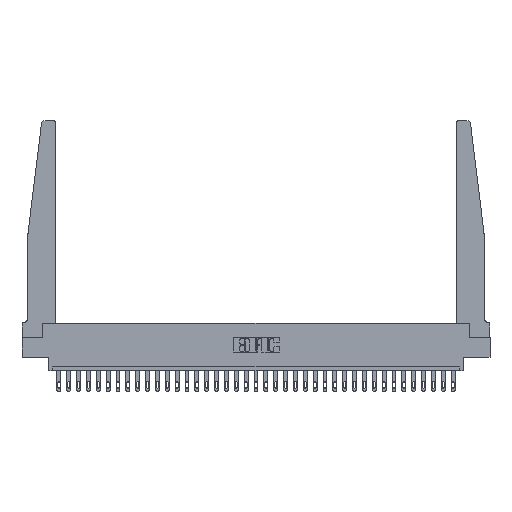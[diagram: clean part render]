
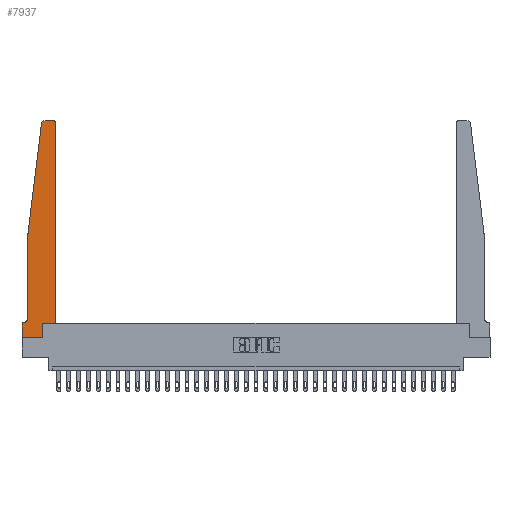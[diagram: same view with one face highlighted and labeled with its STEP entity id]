
A CAD part, top view. The second image highlights one B-rep face of the part: STEP entity #7937.
In plain terms, the highlighted planar face has unit normal (0, 0, 1).
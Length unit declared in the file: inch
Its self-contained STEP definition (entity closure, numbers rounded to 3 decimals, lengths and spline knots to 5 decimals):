
#10 = LINE ( 'NONE', #13769, #247 ) ;
#92 = DIRECTION ( 'NONE',  ( 1., 0., 0. ) ) ;
#103 = LINE ( 'NONE', #4939, #19569 ) ;
#247 = VECTOR ( 'NONE', #9384, 39.37008 ) ;
#401 = CARTESIAN_POINT ( 'NONE',  ( 0., 0.1875, 0.37 ) ) ;
#1106 = VERTEX_POINT ( 'NONE', #29358 ) ;
#1212 = ORIENTED_EDGE ( 'NONE', *, *, #13531, .T. ) ;
#1813 = VERTEX_POINT ( 'NONE', #18830 ) ;
#2293 = FACE_OUTER_BOUND ( 'NONE', #19335, .T. ) ;
#2329 = DIRECTION ( 'NONE',  ( -1., 0., 0. ) ) ;
#2357 = VERTEX_POINT ( 'NONE', #26692 ) ;
#2729 = DIRECTION ( 'NONE',  ( 0., 0., 1. ) ) ;
#2940 = VERTEX_POINT ( 'NONE', #24924 ) ;
#3674 = LINE ( 'NONE', #18184, #15856 ) ;
#3904 = CARTESIAN_POINT ( 'NONE',  ( 0.065, 1.25, 0.37 ) ) ;
#3967 = EDGE_CURVE ( 'NONE', #2940, #1813, #29030, .T. ) ;
#4042 = VECTOR ( 'NONE', #6650, 39.37008 ) ;
#4383 = EDGE_CURVE ( 'NONE', #9635, #28857, #103, .T. ) ;
#4545 = ORIENTED_EDGE ( 'NONE', *, *, #13422, .T. ) ;
#4939 = CARTESIAN_POINT ( 'NONE',  ( 0., 0., 0.37 ) ) ;
#5403 = LINE ( 'NONE', #29280, #7797 ) ;
#5461 = LINE ( 'NONE', #29186, #5809 ) ;
#5809 = VECTOR ( 'NONE', #27000, 39.37008 ) ;
#5812 = VERTEX_POINT ( 'NONE', #6454 ) ;
#6262 = ORIENTED_EDGE ( 'NONE', *, *, #21996, .T. ) ;
#6454 = CARTESIAN_POINT ( 'NONE',  ( 0.015, 0.1875, 0.37 ) ) ;
#6650 = DIRECTION ( 'NONE',  ( 0., 1., 0. ) ) ;
#7498 = DIRECTION ( 'NONE',  ( 0., 0., -1. ) ) ;
#7726 = LINE ( 'NONE', #17232, #14847 ) ;
#7797 = VECTOR ( 'NONE', #22091, 39.37008 ) ;
#7937 = ADVANCED_FACE ( 'NONE', ( #2293 ), #14307, .T. ) ;
#8455 = DIRECTION ( 'NONE',  ( 1., 0., 0. ) ) ;
#8988 = EDGE_CURVE ( 'NONE', #5812, #23784, #5461, .T. ) ;
#9278 = AXIS2_PLACEMENT_3D ( 'NONE', #401, #2729, #92 ) ;
#9384 = DIRECTION ( 'NONE',  ( 0., -1., 0. ) ) ;
#9620 = CARTESIAN_POINT ( 'NONE',  ( 0., 0., 0.37 ) ) ;
#9635 = VERTEX_POINT ( 'NONE', #9620 ) ;
#9976 = CARTESIAN_POINT ( 'NONE',  ( 0.015, 0.2375, 0.37 ) ) ;
#10148 = DIRECTION ( 'NONE',  ( 1., 0., 0. ) ) ;
#10258 = ORIENTED_EDGE ( 'NONE', *, *, #26736, .T. ) ;
#10427 = VERTEX_POINT ( 'NONE', #28549 ) ;
#10448 = ORIENTED_EDGE ( 'NONE', *, *, #3967, .T. ) ;
#10790 = CARTESIAN_POINT ( 'NONE',  ( 0.27653, 2.72, 0.37 ) ) ;
#12201 = ORIENTED_EDGE ( 'NONE', *, *, #4383, .T. ) ;
#12668 = VERTEX_POINT ( 'NONE', #15807 ) ;
#13422 = EDGE_CURVE ( 'NONE', #23784, #9635, #10, .T. ) ;
#13514 = CARTESIAN_POINT ( 'NONE',  ( 0.425, 0.18, 0.37 ) ) ;
#13531 = EDGE_CURVE ( 'NONE', #1106, #5812, #27179, .T. ) ;
#13600 = ORIENTED_EDGE ( 'NONE', *, *, #23601, .T. ) ;
#13769 = CARTESIAN_POINT ( 'NONE',  ( 0., 0., 0.37 ) ) ;
#13875 = EDGE_CURVE ( 'NONE', #1813, #23651, #23681, .T. ) ;
#14013 = DIRECTION ( 'NONE',  ( 1., 0., 0. ) ) ;
#14192 = CARTESIAN_POINT ( 'NONE',  ( 0.25, 2.75, 0.37 ) ) ;
#14307 = PLANE ( 'NONE',  #9278 ) ;
#14679 = VECTOR ( 'NONE', #2329, 39.37008 ) ;
#14847 = VECTOR ( 'NONE', #17072, 39.37008 ) ;
#14982 = CIRCLE ( 'NONE', #29922, 0.03 ) ;
#15807 = CARTESIAN_POINT ( 'NONE',  ( 0.2605, 0.18, 0.37 ) ) ;
#15856 = VECTOR ( 'NONE', #20822, 39.37008 ) ;
#16469 = VECTOR ( 'NONE', #17798, 39.37008 ) ;
#16712 = DIRECTION ( 'NONE',  ( 0., 0., 1. ) ) ;
#17072 = DIRECTION ( 'NONE',  ( 0., 1., 0. ) ) ;
#17232 = CARTESIAN_POINT ( 'NONE',  ( 0.2605, 0.18, 0.37 ) ) ;
#17532 = CARTESIAN_POINT ( 'NONE',  ( 0.27653, 2.75, 0.37 ) ) ;
#17798 = DIRECTION ( 'NONE',  ( 0., -1., 0. ) ) ;
#18184 = CARTESIAN_POINT ( 'NONE',  ( 0.425, 0.18, 0.37 ) ) ;
#18232 = ORIENTED_EDGE ( 'NONE', *, *, #27138, .T. ) ;
#18830 = CARTESIAN_POINT ( 'NONE',  ( 0.395, 2.75, 0.37 ) ) ;
#19335 = EDGE_LOOP ( 'NONE', ( #25082, #10258, #6262, #27633, #1212, #28051, #4545, #12201, #13600, #23103, #18232, #10448 ) ) ;
#19569 = VECTOR ( 'NONE', #14013, 39.37008 ) ;
#20822 = DIRECTION ( 'NONE',  ( 1., 0., 0. ) ) ;
#21899 = VERTEX_POINT ( 'NONE', #26937 ) ;
#21996 = EDGE_CURVE ( 'NONE', #21899, #10427, #5403, .T. ) ;
#22091 = DIRECTION ( 'NONE',  ( -0.122, -0.992, 0. ) ) ;
#22180 = EDGE_CURVE ( 'NONE', #12668, #2357, #3674, .T. ) ;
#22565 = AXIS2_PLACEMENT_3D ( 'NONE', #24332, #16712, #10148 ) ;
#23103 = ORIENTED_EDGE ( 'NONE', *, *, #22180, .T. ) ;
#23131 = CARTESIAN_POINT ( 'NONE',  ( 0., 0.1875, 0.37 ) ) ;
#23601 = EDGE_CURVE ( 'NONE', #28857, #12668, #7726, .T. ) ;
#23651 = VERTEX_POINT ( 'NONE', #17532 ) ;
#23681 = LINE ( 'NONE', #14192, #14679 ) ;
#23784 = VERTEX_POINT ( 'NONE', #23131 ) ;
#24332 = CARTESIAN_POINT ( 'NONE',  ( 0.395, 2.72, 0.37 ) ) ;
#24639 = DIRECTION ( 'NONE',  ( -1., 0., 0. ) ) ;
#24924 = CARTESIAN_POINT ( 'NONE',  ( 0.425, 2.72, 0.37 ) ) ;
#25082 = ORIENTED_EDGE ( 'NONE', *, *, #13875, .T. ) ;
#26692 = CARTESIAN_POINT ( 'NONE',  ( 0.425, 0.18, 0.37 ) ) ;
#26736 = EDGE_CURVE ( 'NONE', #23651, #21899, #14982, .T. ) ;
#26743 = EDGE_CURVE ( 'NONE', #10427, #1106, #27333, .T. ) ;
#26937 = CARTESIAN_POINT ( 'NONE',  ( 0.24675, 2.72367, 0.37 ) ) ;
#27000 = DIRECTION ( 'NONE',  ( -1., 0., 0. ) ) ;
#27138 = EDGE_CURVE ( 'NONE', #2357, #2940, #29626, .T. ) ;
#27179 = CIRCLE ( 'NONE', #30680, 0.05 ) ;
#27333 = LINE ( 'NONE', #3904, #16469 ) ;
#27633 = ORIENTED_EDGE ( 'NONE', *, *, #26743, .T. ) ;
#28051 = ORIENTED_EDGE ( 'NONE', *, *, #8988, .T. ) ;
#28549 = CARTESIAN_POINT ( 'NONE',  ( 0.065, 1.25, 0.37 ) ) ;
#28857 = VERTEX_POINT ( 'NONE', #30687 ) ;
#29030 = CIRCLE ( 'NONE', #22565, 0.03 ) ;
#29186 = CARTESIAN_POINT ( 'NONE',  ( 0.065, 0.1875, 0.37 ) ) ;
#29280 = CARTESIAN_POINT ( 'NONE',  ( 0.065, 1.25, 0.37 ) ) ;
#29358 = CARTESIAN_POINT ( 'NONE',  ( 0.065, 0.2375, 0.37 ) ) ;
#29626 = LINE ( 'NONE', #13514, #4042 ) ;
#29922 = AXIS2_PLACEMENT_3D ( 'NONE', #10790, #30125, #8455 ) ;
#30125 = DIRECTION ( 'NONE',  ( 0., 0., 1. ) ) ;
#30680 = AXIS2_PLACEMENT_3D ( 'NONE', #9976, #7498, #24639 ) ;
#30687 = CARTESIAN_POINT ( 'NONE',  ( 0.2605, 0., 0.37 ) ) ;
